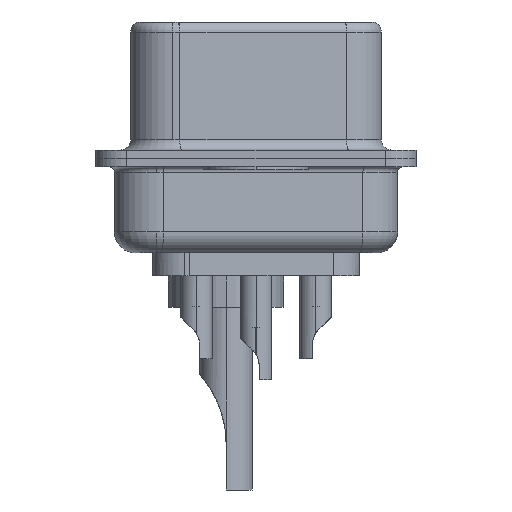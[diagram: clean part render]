
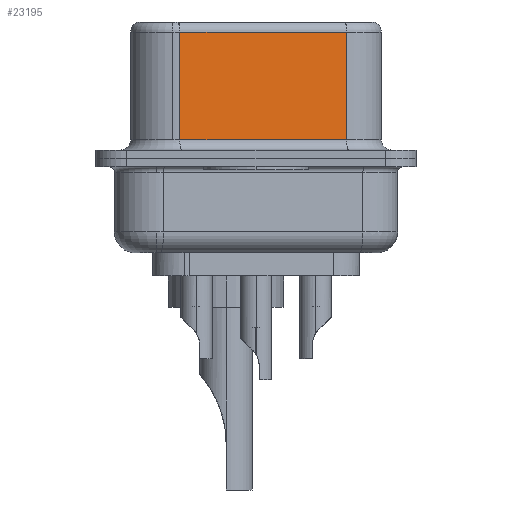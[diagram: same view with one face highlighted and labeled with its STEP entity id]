
A CAD part, left-side view. The second image highlights one B-rep face of the part: STEP entity #23195.
In plain terms, the highlighted planar face has unit normal (-0.985, -0.174, 0).
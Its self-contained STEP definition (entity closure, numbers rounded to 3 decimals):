
#1297 = CARTESIAN_POINT ( 'NONE',  ( 3.73, 3.628, 0.9 ) ) ;
#1875 = VERTEX_POINT ( 'NONE', #15012 ) ;
#2127 = LINE ( 'NONE', #15364, #23510 ) ;
#3246 = LINE ( 'NONE', #24680, #23362 ) ;
#5126 = CARTESIAN_POINT ( 'NONE',  ( 5.132, -4.322, 0.9 ) ) ;
#5265 = LINE ( 'NONE', #5126, #15690 ) ;
#5698 = PLANE ( 'NONE',  #9752 ) ;
#5825 = ORIENTED_EDGE ( 'NONE', *, *, #7973, .T. ) ;
#7198 = DIRECTION ( 'NONE',  ( 0.174, -0.985, 0. ) ) ;
#7771 = DIRECTION ( 'NONE',  ( 0.985, 0.174, 0. ) ) ;
#7973 = EDGE_CURVE ( 'NONE', #1875, #16313, #3246, .T. ) ;
#9752 = AXIS2_PLACEMENT_3D ( 'NONE', #16067, #7771, #22275 ) ;
#10219 = CARTESIAN_POINT ( 'NONE',  ( 5.132, -4.322, 6.02 ) ) ;
#10706 = DIRECTION ( 'NONE',  ( -0.174, 0.985, 0. ) ) ;
#12296 = EDGE_CURVE ( 'NONE', #12535, #14879, #2127, .T. ) ;
#12535 = VERTEX_POINT ( 'NONE', #10219 ) ;
#12932 = LINE ( 'NONE', #21034, #17774 ) ;
#13347 = EDGE_CURVE ( 'NONE', #16313, #14879, #5265, .T. ) ;
#13921 = ORIENTED_EDGE ( 'NONE', *, *, #13347, .T. ) ;
#14585 = ORIENTED_EDGE ( 'NONE', *, *, #20651, .T. ) ;
#14879 = VERTEX_POINT ( 'NONE', #21448 ) ;
#15012 = CARTESIAN_POINT ( 'NONE',  ( 3.73, 3.628, 6.02 ) ) ;
#15364 = CARTESIAN_POINT ( 'NONE',  ( 5.132, -4.322, 6.52 ) ) ;
#15690 = VECTOR ( 'NONE', #7198, 1000. ) ;
#16067 = CARTESIAN_POINT ( 'NONE',  ( 5.132, -4.322, 6.52 ) ) ;
#16313 = VERTEX_POINT ( 'NONE', #1297 ) ;
#17774 = VECTOR ( 'NONE', #10706, 1000. ) ;
#19103 = EDGE_LOOP ( 'NONE', ( #23836, #14585, #5825, #13921 ) ) ;
#20651 = EDGE_CURVE ( 'NONE', #12535, #1875, #12932, .T. ) ;
#21034 = CARTESIAN_POINT ( 'NONE',  ( 5.132, -4.322, 6.02 ) ) ;
#21173 = DIRECTION ( 'NONE',  ( 0., 0., -1. ) ) ;
#21448 = CARTESIAN_POINT ( 'NONE',  ( 5.132, -4.322, 0.9 ) ) ;
#21576 = DIRECTION ( 'NONE',  ( 0., 0., -1. ) ) ;
#22275 = DIRECTION ( 'NONE',  ( -0.174, 0.985, 0. ) ) ;
#23195 = ADVANCED_FACE ( 'NONE', ( #25451 ), #5698, .F. ) ;
#23362 = VECTOR ( 'NONE', #21173, 1000. ) ;
#23510 = VECTOR ( 'NONE', #21576, 1000. ) ;
#23836 = ORIENTED_EDGE ( 'NONE', *, *, #12296, .F. ) ;
#24680 = CARTESIAN_POINT ( 'NONE',  ( 3.73, 3.628, 6.52 ) ) ;
#25451 = FACE_OUTER_BOUND ( 'NONE', #19103, .T. ) ;
